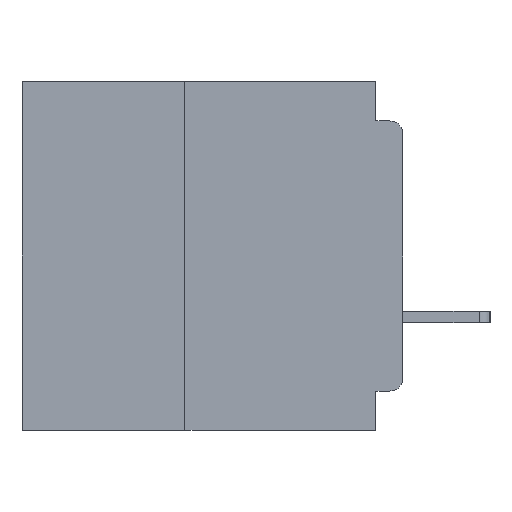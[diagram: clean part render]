
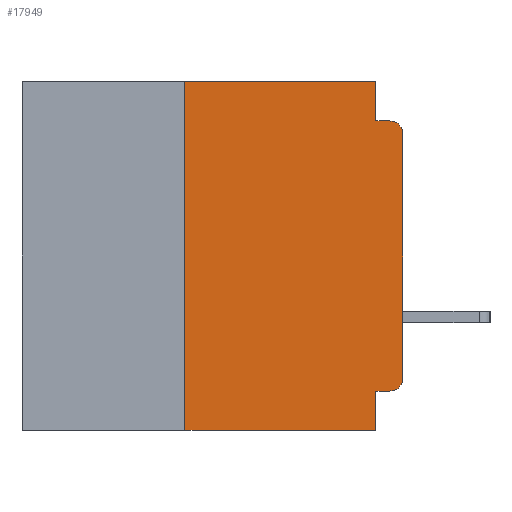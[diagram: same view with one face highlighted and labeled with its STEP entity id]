
A CAD part, left-side view. The second image highlights one B-rep face of the part: STEP entity #17949.
In plain terms, the highlighted planar face has unit normal (-1, 0, 0).
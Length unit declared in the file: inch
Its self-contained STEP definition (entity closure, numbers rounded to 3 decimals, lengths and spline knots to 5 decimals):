
#255 = ORIENTED_EDGE ( 'NONE', *, *, #13027, .F. ) ;
#326 = LINE ( 'NONE', #35009, #24076 ) ;
#378 = ORIENTED_EDGE ( 'NONE', *, *, #12513, .T. ) ;
#563 = DIRECTION ( 'NONE',  ( 0., 0., -1. ) ) ;
#1406 = CIRCLE ( 'NONE', #18841, 0.015 ) ;
#1618 = LINE ( 'NONE', #11658, #11309 ) ;
#1937 = FACE_OUTER_BOUND ( 'NONE', #32120, .T. ) ;
#2597 = VERTEX_POINT ( 'NONE', #17073 ) ;
#3327 = VERTEX_POINT ( 'NONE', #36473 ) ;
#3579 = ORIENTED_EDGE ( 'NONE', *, *, #26568, .T. ) ;
#3827 = CARTESIAN_POINT ( 'NONE',  ( 0., 0.015, -0.34 ) ) ;
#4647 = VERTEX_POINT ( 'NONE', #14334 ) ;
#5441 = CARTESIAN_POINT ( 'NONE',  ( 0., 0., 0. ) ) ;
#7067 = DIRECTION ( 'NONE',  ( 0., 0., -1. ) ) ;
#8674 = CARTESIAN_POINT ( 'NONE',  ( 0., 0.031, -0.355 ) ) ;
#8715 = DIRECTION ( 'NONE',  ( 0., 0., 1. ) ) ;
#8842 = CARTESIAN_POINT ( 'NONE',  ( 0., 0.437, -0.4 ) ) ;
#11309 = VECTOR ( 'NONE', #30669, 39.37008 ) ;
#11658 = CARTESIAN_POINT ( 'NONE',  ( 0., 0.437, 0. ) ) ;
#12477 = CIRCLE ( 'NONE', #22554, 0.015 ) ;
#12513 = EDGE_CURVE ( 'NONE', #14669, #20141, #1406, .T. ) ;
#12804 = AXIS2_PLACEMENT_3D ( 'NONE', #23529, #14018, #36088 ) ;
#13027 = EDGE_CURVE ( 'NONE', #30277, #16690, #326, .T. ) ;
#13783 = VECTOR ( 'NONE', #19821, 39.37008 ) ;
#14018 = DIRECTION ( 'NONE',  ( 1., 0., 0. ) ) ;
#14334 = CARTESIAN_POINT ( 'NONE',  ( 0., 0.25, 0. ) ) ;
#14669 = VERTEX_POINT ( 'NONE', #40452 ) ;
#15745 = CARTESIAN_POINT ( 'NONE',  ( 0., 0.031, -0.4 ) ) ;
#16355 = EDGE_CURVE ( 'NONE', #27225, #21295, #38896, .T. ) ;
#16530 = ORIENTED_EDGE ( 'NONE', *, *, #29383, .F. ) ;
#16563 = CARTESIAN_POINT ( 'NONE',  ( 0., 0., -0.355 ) ) ;
#16690 = VERTEX_POINT ( 'NONE', #33893 ) ;
#17073 = CARTESIAN_POINT ( 'NONE',  ( 0., 0.25, -0.4 ) ) ;
#17949 = ADVANCED_FACE ( 'NONE', ( #1937 ), #32946, .F. ) ;
#18841 = AXIS2_PLACEMENT_3D ( 'NONE', #38705, #20012, #563 ) ;
#18998 = DIRECTION ( 'NONE',  ( 0., 0., -1. ) ) ;
#19746 = VERTEX_POINT ( 'NONE', #20387 ) ;
#19821 = DIRECTION ( 'NONE',  ( 0., 1., 0. ) ) ;
#20012 = DIRECTION ( 'NONE',  ( -1., 0., 0. ) ) ;
#20141 = VERTEX_POINT ( 'NONE', #25555 ) ;
#20387 = CARTESIAN_POINT ( 'NONE',  ( 0., 0., -0.34 ) ) ;
#21295 = VERTEX_POINT ( 'NONE', #8674 ) ;
#21519 = DIRECTION ( 'NONE',  ( 0., -1., 0. ) ) ;
#22554 = AXIS2_PLACEMENT_3D ( 'NONE', #3827, #26252, #7067 ) ;
#23144 = EDGE_CURVE ( 'NONE', #21295, #3327, #26113, .T. ) ;
#23529 = CARTESIAN_POINT ( 'NONE',  ( 0., 0.437, 0. ) ) ;
#24076 = VECTOR ( 'NONE', #31858, 39.37008 ) ;
#24365 = VECTOR ( 'NONE', #8715, 39.37008 ) ;
#24674 = CARTESIAN_POINT ( 'NONE',  ( 0., 0., -0.045 ) ) ;
#24680 = LINE ( 'NONE', #8842, #32983 ) ;
#24833 = DIRECTION ( 'NONE',  ( 0., -1., 0. ) ) ;
#25139 = VECTOR ( 'NONE', #18998, 39.37008 ) ;
#25555 = CARTESIAN_POINT ( 'NONE',  ( 0., 0.015, -0.045 ) ) ;
#26113 = LINE ( 'NONE', #15745, #25139 ) ;
#26252 = DIRECTION ( 'NONE',  ( -1., 0., 0. ) ) ;
#26486 = VECTOR ( 'NONE', #31016, 39.37008 ) ;
#26568 = EDGE_CURVE ( 'NONE', #19746, #14669, #40939, .T. ) ;
#27225 = VERTEX_POINT ( 'NONE', #34331 ) ;
#28410 = EDGE_CURVE ( 'NONE', #2597, #3327, #24680, .T. ) ;
#29383 = EDGE_CURVE ( 'NONE', #4647, #30277, #1618, .T. ) ;
#29894 = VECTOR ( 'NONE', #21519, 39.37008 ) ;
#30277 = VERTEX_POINT ( 'NONE', #38218 ) ;
#30584 = ORIENTED_EDGE ( 'NONE', *, *, #37245, .F. ) ;
#30669 = DIRECTION ( 'NONE',  ( 0., -1., 0. ) ) ;
#30860 = LINE ( 'NONE', #24674, #29894 ) ;
#31016 = DIRECTION ( 'NONE',  ( 0., 0., 1. ) ) ;
#31797 = ORIENTED_EDGE ( 'NONE', *, *, #33605, .T. ) ;
#31858 = DIRECTION ( 'NONE',  ( 0., 0., -1. ) ) ;
#32120 = EDGE_LOOP ( 'NONE', ( #3579, #378, #30584, #255, #16530, #36793, #36401, #34687, #38892, #31797 ) ) ;
#32946 = PLANE ( 'NONE',  #12804 ) ;
#32983 = VECTOR ( 'NONE', #24833, 39.37008 ) ;
#33605 = EDGE_CURVE ( 'NONE', #27225, #19746, #12477, .T. ) ;
#33893 = CARTESIAN_POINT ( 'NONE',  ( 0., 0.031, -0.045 ) ) ;
#34331 = CARTESIAN_POINT ( 'NONE',  ( 0., 0.015, -0.355 ) ) ;
#34687 = ORIENTED_EDGE ( 'NONE', *, *, #23144, .F. ) ;
#34778 = LINE ( 'NONE', #40281, #26486 ) ;
#35009 = CARTESIAN_POINT ( 'NONE',  ( 0., 0.031, 0. ) ) ;
#36088 = DIRECTION ( 'NONE',  ( 0., 0., -1. ) ) ;
#36401 = ORIENTED_EDGE ( 'NONE', *, *, #28410, .T. ) ;
#36473 = CARTESIAN_POINT ( 'NONE',  ( 0., 0.031, -0.4 ) ) ;
#36793 = ORIENTED_EDGE ( 'NONE', *, *, #41236, .F. ) ;
#37245 = EDGE_CURVE ( 'NONE', #16690, #20141, #30860, .T. ) ;
#38218 = CARTESIAN_POINT ( 'NONE',  ( 0., 0.031, 0. ) ) ;
#38705 = CARTESIAN_POINT ( 'NONE',  ( 0., 0.015, -0.06 ) ) ;
#38892 = ORIENTED_EDGE ( 'NONE', *, *, #16355, .F. ) ;
#38896 = LINE ( 'NONE', #16563, #13783 ) ;
#40281 = CARTESIAN_POINT ( 'NONE',  ( 0., 0.25, -0.4 ) ) ;
#40452 = CARTESIAN_POINT ( 'NONE',  ( 0., 0., -0.06 ) ) ;
#40939 = LINE ( 'NONE', #5441, #24365 ) ;
#41236 = EDGE_CURVE ( 'NONE', #2597, #4647, #34778, .T. ) ;
